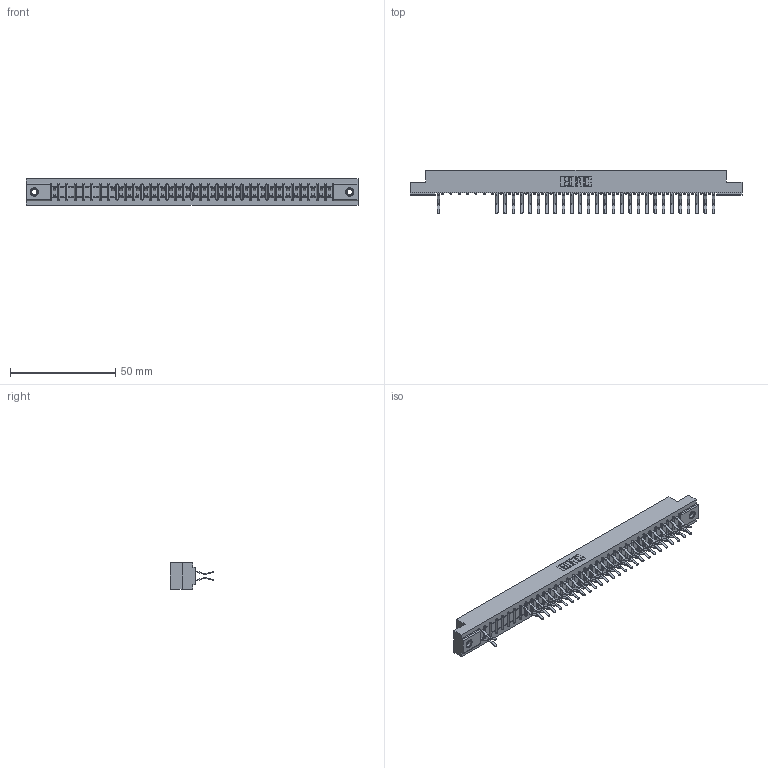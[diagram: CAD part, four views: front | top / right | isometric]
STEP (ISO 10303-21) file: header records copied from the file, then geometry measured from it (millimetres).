
FILE_DESCRIPTION (( 'STEP AP203' ), '1' );
FILE_NAME ('307-068-560-207.STEP', '2018-08-06T12:32:09', ( '' ), ( '' ), 'SwSTEP 2.0', 'SolidWorks 2016', '' );
FILE_SCHEMA (( 'CONFIG_CONTROL_DESIGN' ));
Length unit declared in the file: inch
Products named in the file (4): 307 Part_.156 Dia Mounting Holes; 307-290-001_560; 345-250-001_345-250-005-103; 307-068-560-207
Assembly tree (58 placements, depth 2):
  307-068-560-207
    307 Part_.156 Dia Mounting Holes
    307-290-001_560  x55
    345-250-001_345-250-005-103  x2
Bounding box: 157.73 x 20.73 x 12.7 mm (x, y, z)
Volume: 16603.2 mm3; surface area: 19450.5 mm2
Topology: 58 solids, 58 shells, 3093 faces, 8685 edges, 5614 vertices
Faces by surface type: plane 1995, cylinder 1012, sphere 70, cone 12, torus 4
Entity records: 32095 total; most frequent: CARTESIAN_POINT 5292, ORIENTED_EDGE 5250, DIRECTION 5183, EDGE_CURVE 2625, LINE 2009, VECTOR 2009, VERTEX_POINT 1696, AXIS2_PLACEMENT_3D 1587
